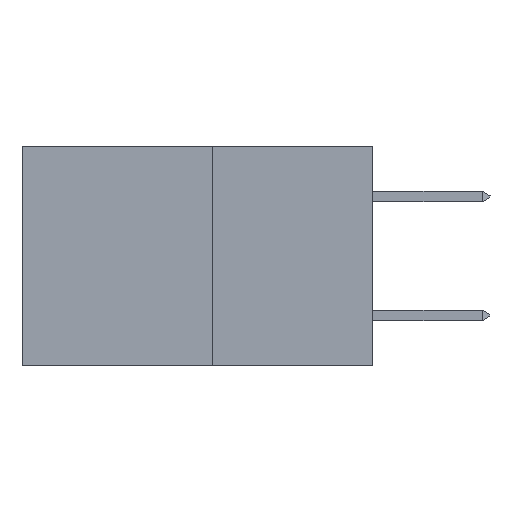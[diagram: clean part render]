
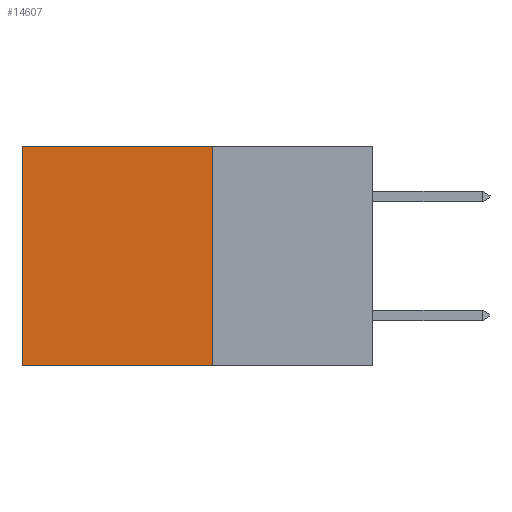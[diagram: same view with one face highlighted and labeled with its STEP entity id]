
A CAD part, left-side view. The second image highlights one B-rep face of the part: STEP entity #14607.
In plain terms, the highlighted planar face has unit normal (-1, 0, 0).
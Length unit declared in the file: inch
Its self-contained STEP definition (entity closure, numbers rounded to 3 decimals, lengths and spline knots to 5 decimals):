
#2099 = CARTESIAN_POINT ( 'NONE',  ( 0.277, 0.27, -0.37 ) ) ;
#2181 = ORIENTED_EDGE ( 'NONE', *, *, #15620, .F. ) ;
#2405 = LINE ( 'NONE', #19312, #14591 ) ;
#2672 = ORIENTED_EDGE ( 'NONE', *, *, #9038, .F. ) ;
#2896 = EDGE_CURVE ( 'NONE', #11650, #12765, #15973, .T. ) ;
#2990 = LINE ( 'NONE', #2099, #10776 ) ;
#3004 = LINE ( 'NONE', #6569, #19305 ) ;
#3501 = CARTESIAN_POINT ( 'NONE',  ( 0.277, 0.59, 0. ) ) ;
#3983 = VERTEX_POINT ( 'NONE', #17125 ) ;
#4155 = CARTESIAN_POINT ( 'NONE',  ( 0.277, 0.59, -0.37 ) ) ;
#4204 = DIRECTION ( 'NONE',  ( 0., 0., -1. ) ) ;
#5954 = EDGE_CURVE ( 'NONE', #19643, #11650, #3004, .T. ) ;
#6569 = CARTESIAN_POINT ( 'NONE',  ( 0.277, 0.27, 0. ) ) ;
#6641 = PLANE ( 'NONE',  #17926 ) ;
#8187 = DIRECTION ( 'NONE',  ( 1., 0., 0. ) ) ;
#8775 = CARTESIAN_POINT ( 'NONE',  ( 0.277, 0.27, 0. ) ) ;
#9038 = EDGE_CURVE ( 'NONE', #19643, #3983, #2405, .T. ) ;
#10204 = DIRECTION ( 'NONE',  ( 0., 1., 0. ) ) ;
#10776 = VECTOR ( 'NONE', #14306, 39.37008 ) ;
#11650 = VERTEX_POINT ( 'NONE', #3501 ) ;
#12048 = ORIENTED_EDGE ( 'NONE', *, *, #2896, .T. ) ;
#12303 = EDGE_LOOP ( 'NONE', ( #12048, #2181, #2672, #12488 ) ) ;
#12436 = VECTOR ( 'NONE', #4204, 39.37008 ) ;
#12488 = ORIENTED_EDGE ( 'NONE', *, *, #5954, .T. ) ;
#12765 = VERTEX_POINT ( 'NONE', #13013 ) ;
#13013 = CARTESIAN_POINT ( 'NONE',  ( 0.277, 0.59, -0.37 ) ) ;
#14306 = DIRECTION ( 'NONE',  ( 0., 1., 0. ) ) ;
#14591 = VECTOR ( 'NONE', #19062, 39.37008 ) ;
#14607 = ADVANCED_FACE ( 'NONE', ( #16624 ), #6641, .F. ) ;
#15620 = EDGE_CURVE ( 'NONE', #3983, #12765, #2990, .T. ) ;
#15973 = LINE ( 'NONE', #4155, #12436 ) ;
#16624 = FACE_OUTER_BOUND ( 'NONE', #12303, .T. ) ;
#17125 = CARTESIAN_POINT ( 'NONE',  ( 0.277, 0.27, -0.37 ) ) ;
#17926 = AXIS2_PLACEMENT_3D ( 'NONE', #18687, #8187, #18760 ) ;
#18687 = CARTESIAN_POINT ( 'NONE',  ( 0.277, 0.27, -0.37 ) ) ;
#18760 = DIRECTION ( 'NONE',  ( 0., 0., -1. ) ) ;
#19062 = DIRECTION ( 'NONE',  ( 0., 0., -1. ) ) ;
#19305 = VECTOR ( 'NONE', #10204, 39.37008 ) ;
#19312 = CARTESIAN_POINT ( 'NONE',  ( 0.277, 0.27, -0.37 ) ) ;
#19643 = VERTEX_POINT ( 'NONE', #8775 ) ;
